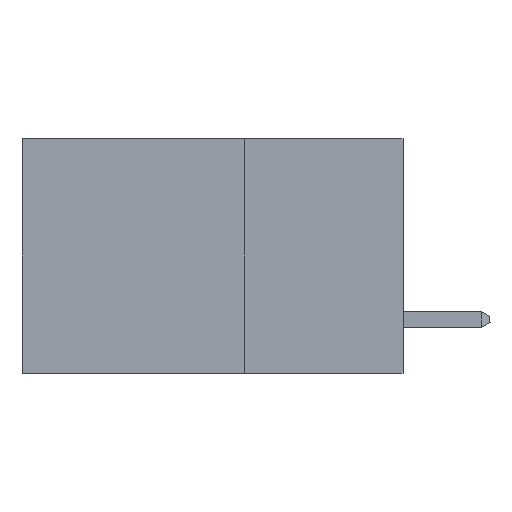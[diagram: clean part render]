
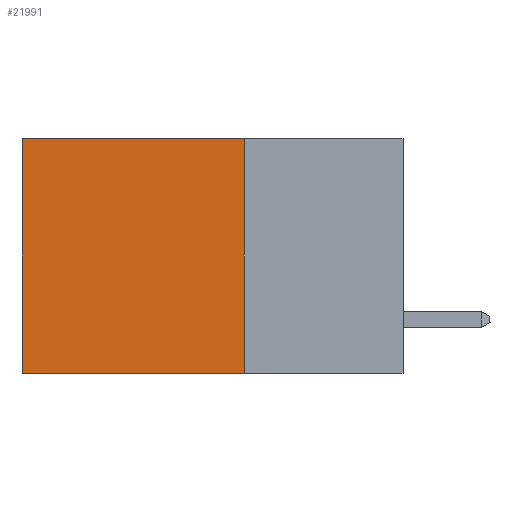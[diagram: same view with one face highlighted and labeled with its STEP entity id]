
A CAD part, left-side view. The second image highlights one B-rep face of the part: STEP entity #21991.
In plain terms, the highlighted planar face has unit normal (-1, 0, 0).
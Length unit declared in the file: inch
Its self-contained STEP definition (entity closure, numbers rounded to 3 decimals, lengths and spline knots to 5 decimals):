
#181 = PLANE ( 'NONE',  #395 ) ;
#395 = AXIS2_PLACEMENT_3D ( 'NONE', #1907, #5425, #15879 ) ;
#807 = FACE_OUTER_BOUND ( 'NONE', #3752, .T. ) ;
#905 = DIRECTION ( 'NONE',  ( 0., 1., 0. ) ) ;
#1375 = CARTESIAN_POINT ( 'NONE',  ( 0.2875, 0.25, -0.37 ) ) ;
#1532 = DIRECTION ( 'NONE',  ( 0., 0., -1. ) ) ;
#1907 = CARTESIAN_POINT ( 'NONE',  ( 0.2875, 0.25, 0. ) ) ;
#2497 = CARTESIAN_POINT ( 'NONE',  ( 0.2875, 0.25, -0.37 ) ) ;
#2630 = VERTEX_POINT ( 'NONE', #22080 ) ;
#2827 = VERTEX_POINT ( 'NONE', #11835 ) ;
#3752 = EDGE_LOOP ( 'NONE', ( #16549, #14202, #8997, #6543 ) ) ;
#5425 = DIRECTION ( 'NONE',  ( 1., 0., 0. ) ) ;
#5887 = EDGE_CURVE ( 'NONE', #16029, #19684, #16438, .T. ) ;
#5906 = DIRECTION ( 'NONE',  ( 0., 1., 0. ) ) ;
#6046 = DIRECTION ( 'NONE',  ( 0., 0., -1. ) ) ;
#6543 = ORIENTED_EDGE ( 'NONE', *, *, #17035, .T. ) ;
#8165 = VECTOR ( 'NONE', #1532, 39.37008 ) ;
#8997 = ORIENTED_EDGE ( 'NONE', *, *, #5887, .F. ) ;
#10562 = VECTOR ( 'NONE', #905, 39.37008 ) ;
#11100 = LINE ( 'NONE', #2497, #10562 ) ;
#11580 = VECTOR ( 'NONE', #6046, 39.37008 ) ;
#11668 = CARTESIAN_POINT ( 'NONE',  ( 0.2875, 0.6, 0. ) ) ;
#11835 = CARTESIAN_POINT ( 'NONE',  ( 0.2875, 0.6, 0. ) ) ;
#12478 = EDGE_CURVE ( 'NONE', #2827, #2630, #13822, .T. ) ;
#13221 = EDGE_CURVE ( 'NONE', #19684, #2630, #11100, .T. ) ;
#13822 = LINE ( 'NONE', #11668, #8165 ) ;
#14202 = ORIENTED_EDGE ( 'NONE', *, *, #13221, .F. ) ;
#15230 = CARTESIAN_POINT ( 'NONE',  ( 0.2875, 0.25, 0. ) ) ;
#15879 = DIRECTION ( 'NONE',  ( 0., 0., -1. ) ) ;
#16029 = VERTEX_POINT ( 'NONE', #15230 ) ;
#16438 = LINE ( 'NONE', #21689, #11580 ) ;
#16549 = ORIENTED_EDGE ( 'NONE', *, *, #12478, .T. ) ;
#17035 = EDGE_CURVE ( 'NONE', #16029, #2827, #17274, .T. ) ;
#17274 = LINE ( 'NONE', #19790, #18373 ) ;
#18373 = VECTOR ( 'NONE', #5906, 39.37008 ) ;
#19684 = VERTEX_POINT ( 'NONE', #1375 ) ;
#19790 = CARTESIAN_POINT ( 'NONE',  ( 0.2875, 0.25, 0. ) ) ;
#21689 = CARTESIAN_POINT ( 'NONE',  ( 0.2875, 0.25, 0. ) ) ;
#21991 = ADVANCED_FACE ( 'NONE', ( #807 ), #181, .F. ) ;
#22080 = CARTESIAN_POINT ( 'NONE',  ( 0.2875, 0.6, -0.37 ) ) ;
